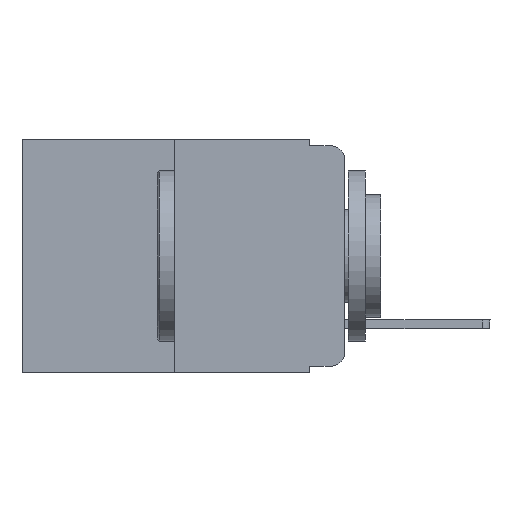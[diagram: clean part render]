
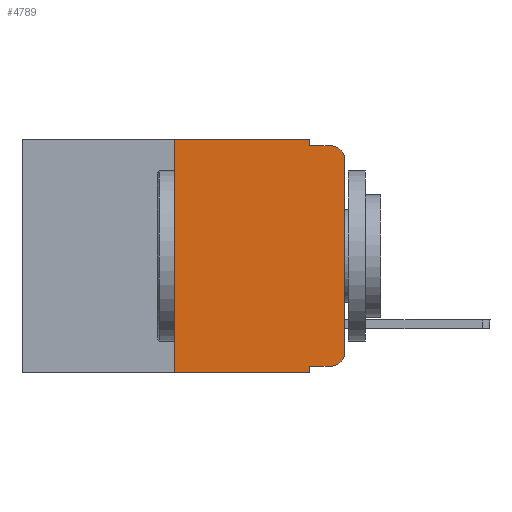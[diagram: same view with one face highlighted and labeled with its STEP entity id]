
A CAD part, left-side view. The second image highlights one B-rep face of the part: STEP entity #4789.
In plain terms, the highlighted planar face has unit normal (-1, 0, 0).
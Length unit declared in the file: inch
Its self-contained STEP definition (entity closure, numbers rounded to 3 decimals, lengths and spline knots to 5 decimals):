
#384 = VECTOR ( 'NONE', #8895, 39.37008 ) ;
#474 = CARTESIAN_POINT ( 'NONE',  ( 0., 0.051, -0.01 ) ) ;
#704 = DIRECTION ( 'NONE',  ( 0., -1., 0. ) ) ;
#747 = CARTESIAN_POINT ( 'NONE',  ( 0., 0., -0.313 ) ) ;
#797 = CIRCLE ( 'NONE', #21392, 0.02 ) ;
#817 = CARTESIAN_POINT ( 'NONE',  ( 0., 0.02, -0.01 ) ) ;
#1105 = DIRECTION ( 'NONE',  ( 0., 0., -1. ) ) ;
#1286 = DIRECTION ( 'NONE',  ( 0., -1., 0. ) ) ;
#1398 = AXIS2_PLACEMENT_3D ( 'NONE', #13920, #18801, #11870 ) ;
#1450 = DIRECTION ( 'NONE',  ( -1., 0., 0. ) ) ;
#1519 = CARTESIAN_POINT ( 'NONE',  ( 0., 0.051, -0.01 ) ) ;
#1597 = FACE_OUTER_BOUND ( 'NONE', #19489, .T. ) ;
#1659 = VERTEX_POINT ( 'NONE', #817 ) ;
#1720 = EDGE_CURVE ( 'NONE', #5426, #1659, #7493, .T. ) ;
#1992 = LINE ( 'NONE', #10357, #384 ) ;
#2146 = DIRECTION ( 'NONE',  ( -1., 0., 0. ) ) ;
#2504 = LINE ( 'NONE', #11423, #6691 ) ;
#3302 = LINE ( 'NONE', #11549, #5471 ) ;
#3332 = LINE ( 'NONE', #10328, #15633 ) ;
#3396 = PLANE ( 'NONE',  #1398 ) ;
#3407 = VECTOR ( 'NONE', #6528, 39.37008 ) ;
#3432 = EDGE_CURVE ( 'NONE', #21058, #11302, #1992, .T. ) ;
#3759 = DIRECTION ( 'NONE',  ( 0., 0., 1. ) ) ;
#3840 = DIRECTION ( 'NONE',  ( 0., 0., -1. ) ) ;
#4789 = ADVANCED_FACE ( 'NONE', ( #1597 ), #3396, .F. ) ;
#4961 = EDGE_CURVE ( 'NONE', #15695, #9389, #13663, .T. ) ;
#5166 = LINE ( 'NONE', #19297, #19390 ) ;
#5222 = ORIENTED_EDGE ( 'NONE', *, *, #13538, .T. ) ;
#5426 = VERTEX_POINT ( 'NONE', #1519 ) ;
#5471 = VECTOR ( 'NONE', #1286, 39.37008 ) ;
#5925 = VERTEX_POINT ( 'NONE', #13484 ) ;
#6504 = CARTESIAN_POINT ( 'NONE',  ( 0., 0.051, -0.343 ) ) ;
#6528 = DIRECTION ( 'NONE',  ( 0., 0., -1. ) ) ;
#6666 = EDGE_CURVE ( 'NONE', #14897, #5426, #21569, .T. ) ;
#6691 = VECTOR ( 'NONE', #20042, 39.37008 ) ;
#7185 = VECTOR ( 'NONE', #704, 39.37008 ) ;
#7231 = ORIENTED_EDGE ( 'NONE', *, *, #17613, .F. ) ;
#7493 = LINE ( 'NONE', #474, #7185 ) ;
#8703 = ORIENTED_EDGE ( 'NONE', *, *, #14188, .T. ) ;
#8895 = DIRECTION ( 'NONE',  ( 0., 0., -1. ) ) ;
#9389 = VERTEX_POINT ( 'NONE', #747 ) ;
#9948 = VERTEX_POINT ( 'NONE', #21538 ) ;
#10239 = ORIENTED_EDGE ( 'NONE', *, *, #3432, .F. ) ;
#10256 = CARTESIAN_POINT ( 'NONE',  ( 0., 0.051, 0. ) ) ;
#10328 = CARTESIAN_POINT ( 'NONE',  ( 0., 0.473, -0.343 ) ) ;
#10336 = DIRECTION ( 'NONE',  ( 0., 0., 1. ) ) ;
#10357 = CARTESIAN_POINT ( 'NONE',  ( 0., 0.051, 0. ) ) ;
#10794 = CARTESIAN_POINT ( 'NONE',  ( 0., 0.051, -0.333 ) ) ;
#10989 = CARTESIAN_POINT ( 'NONE',  ( 0., 0.25, 0. ) ) ;
#11302 = VERTEX_POINT ( 'NONE', #6504 ) ;
#11423 = CARTESIAN_POINT ( 'NONE',  ( 0., 0.473, 0. ) ) ;
#11425 = VERTEX_POINT ( 'NONE', #13843 ) ;
#11549 = CARTESIAN_POINT ( 'NONE',  ( 0., 0.051, -0.333 ) ) ;
#11870 = DIRECTION ( 'NONE',  ( 0., 0., -1. ) ) ;
#11918 = DIRECTION ( 'NONE',  ( 0., -1., 0. ) ) ;
#12021 = ORIENTED_EDGE ( 'NONE', *, *, #1720, .F. ) ;
#12675 = EDGE_CURVE ( 'NONE', #21058, #15695, #3302, .T. ) ;
#13423 = CARTESIAN_POINT ( 'NONE',  ( 0., 0.051, 0. ) ) ;
#13484 = CARTESIAN_POINT ( 'NONE',  ( 0., 0., -0.03 ) ) ;
#13538 = EDGE_CURVE ( 'NONE', #5925, #1659, #797, .T. ) ;
#13663 = CIRCLE ( 'NONE', #20896, 0.02 ) ;
#13843 = CARTESIAN_POINT ( 'NONE',  ( 0., 0.25, -0.343 ) ) ;
#13920 = CARTESIAN_POINT ( 'NONE',  ( 0., 0.473, 0. ) ) ;
#14188 = EDGE_CURVE ( 'NONE', #11425, #11302, #3332, .T. ) ;
#14257 = CARTESIAN_POINT ( 'NONE',  ( 0., 0.02, -0.313 ) ) ;
#14897 = VERTEX_POINT ( 'NONE', #10256 ) ;
#15633 = VECTOR ( 'NONE', #11918, 39.37008 ) ;
#15695 = VERTEX_POINT ( 'NONE', #16332 ) ;
#15767 = LINE ( 'NONE', #10989, #17510 ) ;
#16094 = ORIENTED_EDGE ( 'NONE', *, *, #20955, .T. ) ;
#16332 = CARTESIAN_POINT ( 'NONE',  ( 0., 0.02, -0.333 ) ) ;
#17510 = VECTOR ( 'NONE', #3759, 39.37008 ) ;
#17613 = EDGE_CURVE ( 'NONE', #11425, #9948, #15767, .T. ) ;
#17743 = EDGE_CURVE ( 'NONE', #9948, #14897, #2504, .T. ) ;
#17904 = ORIENTED_EDGE ( 'NONE', *, *, #6666, .F. ) ;
#18539 = ORIENTED_EDGE ( 'NONE', *, *, #4961, .T. ) ;
#18801 = DIRECTION ( 'NONE',  ( 1., 0., 0. ) ) ;
#19297 = CARTESIAN_POINT ( 'NONE',  ( 0., 0., 0. ) ) ;
#19390 = VECTOR ( 'NONE', #10336, 39.37008 ) ;
#19489 = EDGE_LOOP ( 'NONE', ( #16094, #5222, #12021, #17904, #19806, #7231, #8703, #10239, #20236, #18539 ) ) ;
#19806 = ORIENTED_EDGE ( 'NONE', *, *, #17743, .F. ) ;
#20001 = CARTESIAN_POINT ( 'NONE',  ( 0., 0.02, -0.03 ) ) ;
#20042 = DIRECTION ( 'NONE',  ( 0., -1., 0. ) ) ;
#20236 = ORIENTED_EDGE ( 'NONE', *, *, #12675, .T. ) ;
#20896 = AXIS2_PLACEMENT_3D ( 'NONE', #14257, #2146, #3840 ) ;
#20955 = EDGE_CURVE ( 'NONE', #9389, #5925, #5166, .T. ) ;
#21058 = VERTEX_POINT ( 'NONE', #10794 ) ;
#21392 = AXIS2_PLACEMENT_3D ( 'NONE', #20001, #1450, #1105 ) ;
#21538 = CARTESIAN_POINT ( 'NONE',  ( 0., 0.25, 0. ) ) ;
#21569 = LINE ( 'NONE', #13423, #3407 ) ;
